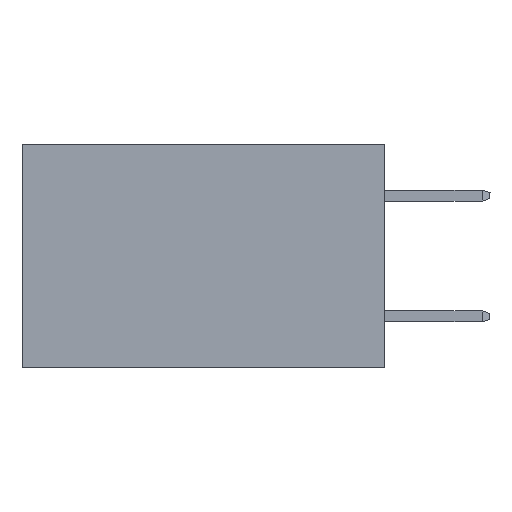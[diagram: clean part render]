
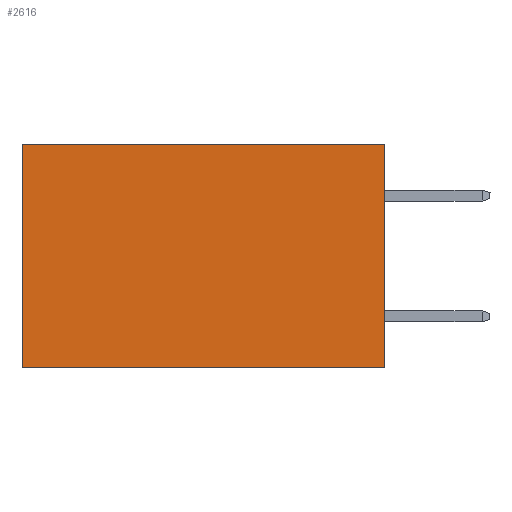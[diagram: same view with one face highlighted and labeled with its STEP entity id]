
A CAD part, left-side view. The second image highlights one B-rep face of the part: STEP entity #2616.
In plain terms, the highlighted planar face has unit normal (-1, 0, 0).
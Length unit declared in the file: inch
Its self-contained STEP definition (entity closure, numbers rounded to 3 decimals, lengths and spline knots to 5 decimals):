
#437 = DIRECTION ( 'NONE',  ( 0., 0., -1. ) ) ;
#460 = EDGE_CURVE ( 'NONE', #5062, #6647, #832, .T. ) ;
#818 = CARTESIAN_POINT ( 'NONE',  ( 0.298, 0.6, 0. ) ) ;
#832 = LINE ( 'NONE', #1686, #8732 ) ;
#1092 = ORIENTED_EDGE ( 'NONE', *, *, #2470, .T. ) ;
#1230 = DIRECTION ( 'NONE',  ( 0., 0., -1. ) ) ;
#1251 = VECTOR ( 'NONE', #4601, 39.37008 ) ;
#1272 = CARTESIAN_POINT ( 'NONE',  ( 0.298, 0., -0.37 ) ) ;
#1287 = EDGE_LOOP ( 'NONE', ( #1092, #5691, #7612, #3361 ) ) ;
#1458 = VECTOR ( 'NONE', #437, 39.37008 ) ;
#1686 = CARTESIAN_POINT ( 'NONE',  ( 0.298, 0., 0. ) ) ;
#2091 = EDGE_CURVE ( 'NONE', #5062, #5462, #3201, .T. ) ;
#2429 = FACE_OUTER_BOUND ( 'NONE', #1287, .T. ) ;
#2470 = EDGE_CURVE ( 'NONE', #6647, #6812, #2544, .T. ) ;
#2544 = LINE ( 'NONE', #3915, #1458 ) ;
#2616 = ADVANCED_FACE ( 'NONE', ( #2429 ), #5527, .F. ) ;
#3201 = LINE ( 'NONE', #6077, #1251 ) ;
#3361 = ORIENTED_EDGE ( 'NONE', *, *, #460, .T. ) ;
#3915 = CARTESIAN_POINT ( 'NONE',  ( 0.298, 0.6, 0. ) ) ;
#4601 = DIRECTION ( 'NONE',  ( 0., 0., -1. ) ) ;
#4724 = CARTESIAN_POINT ( 'NONE',  ( 0.298, 0., -0.37 ) ) ;
#5062 = VERTEX_POINT ( 'NONE', #7227 ) ;
#5462 = VERTEX_POINT ( 'NONE', #4724 ) ;
#5527 = PLANE ( 'NONE',  #8615 ) ;
#5691 = ORIENTED_EDGE ( 'NONE', *, *, #7318, .F. ) ;
#5753 = DIRECTION ( 'NONE',  ( 0., 1., 0. ) ) ;
#6077 = CARTESIAN_POINT ( 'NONE',  ( 0.298, 0., 0. ) ) ;
#6206 = DIRECTION ( 'NONE',  ( 1., 0., 0. ) ) ;
#6214 = DIRECTION ( 'NONE',  ( 0., 1., 0. ) ) ;
#6647 = VERTEX_POINT ( 'NONE', #818 ) ;
#6812 = VERTEX_POINT ( 'NONE', #8952 ) ;
#7227 = CARTESIAN_POINT ( 'NONE',  ( 0.298, 0., 0. ) ) ;
#7318 = EDGE_CURVE ( 'NONE', #5462, #6812, #7334, .T. ) ;
#7334 = LINE ( 'NONE', #1272, #8977 ) ;
#7612 = ORIENTED_EDGE ( 'NONE', *, *, #2091, .F. ) ;
#8615 = AXIS2_PLACEMENT_3D ( 'NONE', #8929, #6206, #1230 ) ;
#8732 = VECTOR ( 'NONE', #5753, 39.37008 ) ;
#8929 = CARTESIAN_POINT ( 'NONE',  ( 0.298, 0., 0. ) ) ;
#8952 = CARTESIAN_POINT ( 'NONE',  ( 0.298, 0.6, -0.37 ) ) ;
#8977 = VECTOR ( 'NONE', #6214, 39.37008 ) ;
